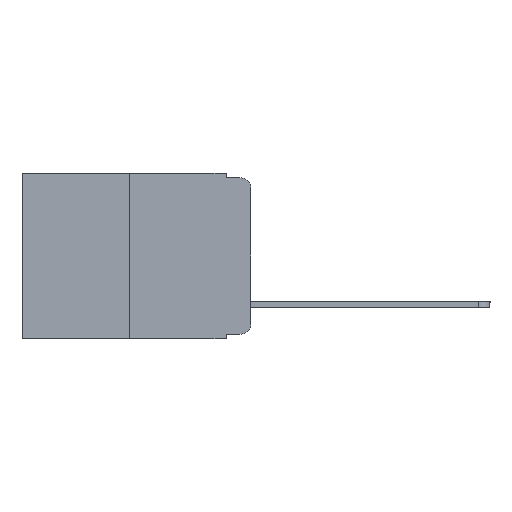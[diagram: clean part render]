
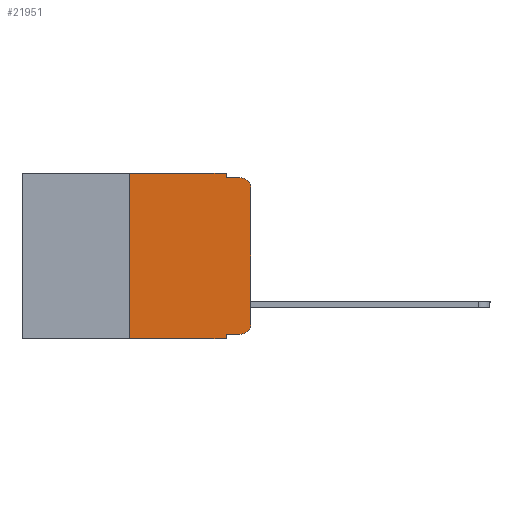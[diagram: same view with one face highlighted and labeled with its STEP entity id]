
A CAD part, left-side view. The second image highlights one B-rep face of the part: STEP entity #21951.
In plain terms, the highlighted planar face has unit normal (-1, 0, 0).
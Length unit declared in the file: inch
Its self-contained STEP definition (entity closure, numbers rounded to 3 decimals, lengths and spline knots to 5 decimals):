
#149 = LINE ( 'NONE', #12091, #17625 ) ;
#195 = CARTESIAN_POINT ( 'NONE',  ( 0., 0., -0.03 ) ) ;
#289 = VERTEX_POINT ( 'NONE', #4737 ) ;
#429 = EDGE_CURVE ( 'NONE', #289, #18048, #149, .T. ) ;
#491 = ORIENTED_EDGE ( 'NONE', *, *, #16678, .F. ) ;
#689 = CARTESIAN_POINT ( 'NONE',  ( 0., 0., 0. ) ) ;
#1140 = CARTESIAN_POINT ( 'NONE',  ( 0., 0., -0.313 ) ) ;
#1147 = CARTESIAN_POINT ( 'NONE',  ( 0., 0.051, 0. ) ) ;
#1157 = DIRECTION ( 'NONE',  ( 0., -1., 0. ) ) ;
#1320 = LINE ( 'NONE', #3102, #21714 ) ;
#1798 = EDGE_CURVE ( 'NONE', #18048, #4101, #19327, .T. ) ;
#2274 = DIRECTION ( 'NONE',  ( 0., 0., 1. ) ) ;
#2639 = ORIENTED_EDGE ( 'NONE', *, *, #20910, .T. ) ;
#2685 = DIRECTION ( 'NONE',  ( 0., 0., 1. ) ) ;
#3102 = CARTESIAN_POINT ( 'NONE',  ( 0., 0.473, -0.343 ) ) ;
#3319 = ORIENTED_EDGE ( 'NONE', *, *, #6428, .F. ) ;
#3670 = CIRCLE ( 'NONE', #5839, 0.02 ) ;
#4101 = VERTEX_POINT ( 'NONE', #14908 ) ;
#4298 = LINE ( 'NONE', #21669, #5396 ) ;
#4476 = CARTESIAN_POINT ( 'NONE',  ( 0., 0.051, 0. ) ) ;
#4507 = CARTESIAN_POINT ( 'NONE',  ( 0., 0.051, -0.333 ) ) ;
#4737 = CARTESIAN_POINT ( 'NONE',  ( 0., 0.25, 0. ) ) ;
#5396 = VECTOR ( 'NONE', #1157, 39.37008 ) ;
#5742 = PLANE ( 'NONE',  #19638 ) ;
#5839 = AXIS2_PLACEMENT_3D ( 'NONE', #18486, #6556, #13696 ) ;
#5873 = CARTESIAN_POINT ( 'NONE',  ( 0., 0.051, -0.01 ) ) ;
#6428 = EDGE_CURVE ( 'NONE', #18395, #289, #10779, .T. ) ;
#6556 = DIRECTION ( 'NONE',  ( -1., 0., 0. ) ) ;
#6815 = ORIENTED_EDGE ( 'NONE', *, *, #429, .F. ) ;
#6820 = ORIENTED_EDGE ( 'NONE', *, *, #21547, .F. ) ;
#6862 = CIRCLE ( 'NONE', #11459, 0.02 ) ;
#6963 = ORIENTED_EDGE ( 'NONE', *, *, #11278, .T. ) ;
#6972 = DIRECTION ( 'NONE',  ( 0., -1., 0. ) ) ;
#7788 = DIRECTION ( 'NONE',  ( -1., 0., 0. ) ) ;
#7834 = EDGE_CURVE ( 'NONE', #17812, #21917, #4298, .T. ) ;
#8152 = DIRECTION ( 'NONE',  ( 0., -1., 0. ) ) ;
#9307 = DIRECTION ( 'NONE',  ( 0., 0., -1. ) ) ;
#9960 = EDGE_CURVE ( 'NONE', #20336, #12938, #6862, .T. ) ;
#10779 = LINE ( 'NONE', #14239, #14251 ) ;
#11027 = CARTESIAN_POINT ( 'NONE',  ( 0., 0.02, -0.01 ) ) ;
#11278 = EDGE_CURVE ( 'NONE', #21917, #12078, #3670, .T. ) ;
#11459 = AXIS2_PLACEMENT_3D ( 'NONE', #16265, #7788, #14594 ) ;
#11933 = ORIENTED_EDGE ( 'NONE', *, *, #7834, .T. ) ;
#12078 = VERTEX_POINT ( 'NONE', #1140 ) ;
#12091 = CARTESIAN_POINT ( 'NONE',  ( 0., 0.473, 0. ) ) ;
#12778 = DIRECTION ( 'NONE',  ( 0., -1., 0. ) ) ;
#12938 = VERTEX_POINT ( 'NONE', #11027 ) ;
#13078 = VECTOR ( 'NONE', #14761, 39.37008 ) ;
#13202 = CARTESIAN_POINT ( 'NONE',  ( 0., 0.051, 0. ) ) ;
#13358 = VECTOR ( 'NONE', #14420, 39.37008 ) ;
#13497 = VECTOR ( 'NONE', #2685, 39.37008 ) ;
#13508 = CARTESIAN_POINT ( 'NONE',  ( 0., 0.25, -0.343 ) ) ;
#13696 = DIRECTION ( 'NONE',  ( 0., 0., -1. ) ) ;
#14182 = ORIENTED_EDGE ( 'NONE', *, *, #9960, .T. ) ;
#14228 = DIRECTION ( 'NONE',  ( 1., 0., 0. ) ) ;
#14239 = CARTESIAN_POINT ( 'NONE',  ( 0., 0.25, 0. ) ) ;
#14251 = VECTOR ( 'NONE', #2274, 39.37008 ) ;
#14321 = LINE ( 'NONE', #689, #13497 ) ;
#14420 = DIRECTION ( 'NONE',  ( 0., 0., -1. ) ) ;
#14594 = DIRECTION ( 'NONE',  ( 0., 0., -1. ) ) ;
#14761 = DIRECTION ( 'NONE',  ( 0., 0., -1. ) ) ;
#14866 = LINE ( 'NONE', #1147, #13078 ) ;
#14908 = CARTESIAN_POINT ( 'NONE',  ( 0., 0.051, -0.01 ) ) ;
#15673 = FACE_OUTER_BOUND ( 'NONE', #19218, .T. ) ;
#15896 = CARTESIAN_POINT ( 'NONE',  ( 0., 0.473, 0. ) ) ;
#16265 = CARTESIAN_POINT ( 'NONE',  ( 0., 0.02, -0.03 ) ) ;
#16678 = EDGE_CURVE ( 'NONE', #17812, #21953, #14866, .T. ) ;
#16899 = CARTESIAN_POINT ( 'NONE',  ( 0., 0.02, -0.333 ) ) ;
#17625 = VECTOR ( 'NONE', #6972, 39.37008 ) ;
#17812 = VERTEX_POINT ( 'NONE', #4507 ) ;
#18048 = VERTEX_POINT ( 'NONE', #13202 ) ;
#18395 = VERTEX_POINT ( 'NONE', #13508 ) ;
#18486 = CARTESIAN_POINT ( 'NONE',  ( 0., 0.02, -0.313 ) ) ;
#19218 = EDGE_LOOP ( 'NONE', ( #21482, #14182, #6820, #20948, #6815, #3319, #2639, #491, #11933, #6963 ) ) ;
#19327 = LINE ( 'NONE', #4476, #13358 ) ;
#19586 = EDGE_CURVE ( 'NONE', #12078, #20336, #14321, .T. ) ;
#19638 = AXIS2_PLACEMENT_3D ( 'NONE', #15896, #14228, #9307 ) ;
#20336 = VERTEX_POINT ( 'NONE', #195 ) ;
#20344 = VECTOR ( 'NONE', #12778, 39.37008 ) ;
#20910 = EDGE_CURVE ( 'NONE', #18395, #21953, #1320, .T. ) ;
#20948 = ORIENTED_EDGE ( 'NONE', *, *, #1798, .F. ) ;
#21008 = CARTESIAN_POINT ( 'NONE',  ( 0., 0.051, -0.343 ) ) ;
#21034 = LINE ( 'NONE', #5873, #20344 ) ;
#21482 = ORIENTED_EDGE ( 'NONE', *, *, #19586, .T. ) ;
#21547 = EDGE_CURVE ( 'NONE', #4101, #12938, #21034, .T. ) ;
#21669 = CARTESIAN_POINT ( 'NONE',  ( 0., 0.051, -0.333 ) ) ;
#21714 = VECTOR ( 'NONE', #8152, 39.37008 ) ;
#21917 = VERTEX_POINT ( 'NONE', #16899 ) ;
#21951 = ADVANCED_FACE ( 'NONE', ( #15673 ), #5742, .F. ) ;
#21953 = VERTEX_POINT ( 'NONE', #21008 ) ;
